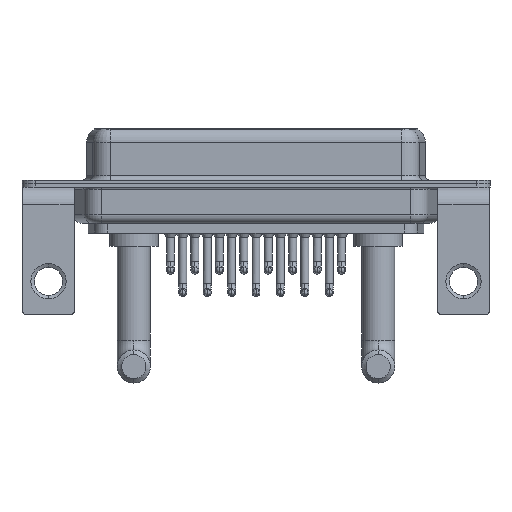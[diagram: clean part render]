
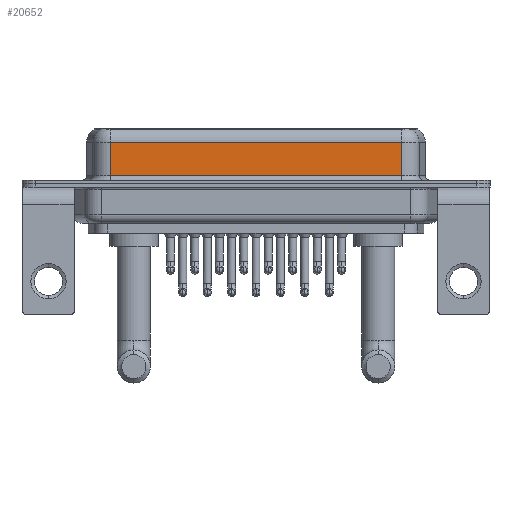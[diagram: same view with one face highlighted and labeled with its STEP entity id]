
A CAD part, front view. The second image highlights one B-rep face of the part: STEP entity #20652.
In plain terms, the highlighted planar face has unit normal (0, -1, 0).
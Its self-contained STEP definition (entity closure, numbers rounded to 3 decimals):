
#88 = DIRECTION ( 'NONE',  ( -1., 0., 0. ) ) ;
#593 = ORIENTED_EDGE ( 'NONE', *, *, #19188, .T. ) ;
#1705 = DIRECTION ( 'NONE',  ( 0., 0., -1. ) ) ;
#2007 = ORIENTED_EDGE ( 'NONE', *, *, #19016, .F. ) ;
#2986 = ORIENTED_EDGE ( 'NONE', *, *, #3895, .T. ) ;
#3107 = EDGE_CURVE ( 'NONE', #15258, #9774, #12984, .T. ) ;
#3604 = VERTEX_POINT ( 'NONE', #16222 ) ;
#3895 = EDGE_CURVE ( 'NONE', #4087, #15258, #15090, .T. ) ;
#4087 = VERTEX_POINT ( 'NONE', #20747 ) ;
#5536 = VECTOR ( 'NONE', #12917, 1000. ) ;
#6944 = VECTOR ( 'NONE', #18664, 1000. ) ;
#7232 = CARTESIAN_POINT ( 'NONE',  ( 7.013, -3.95, 4.65 ) ) ;
#7473 = AXIS2_PLACEMENT_3D ( 'NONE', #18118, #8065, #13878 ) ;
#8065 = DIRECTION ( 'NONE',  ( 0., 1., 0. ) ) ;
#8411 = CARTESIAN_POINT ( 'NONE',  ( 40.037, -3.95, 4.65 ) ) ;
#8516 = LINE ( 'NONE', #13898, #6944 ) ;
#9628 = LINE ( 'NONE', #14343, #5536 ) ;
#9713 = FACE_OUTER_BOUND ( 'NONE', #12321, .T. ) ;
#9774 = VERTEX_POINT ( 'NONE', #10964 ) ;
#10964 = CARTESIAN_POINT ( 'NONE',  ( 7.013, -3.95, 0.9 ) ) ;
#11774 = ORIENTED_EDGE ( 'NONE', *, *, #3107, .T. ) ;
#12321 = EDGE_LOOP ( 'NONE', ( #2007, #2986, #11774, #593 ) ) ;
#12917 = DIRECTION ( 'NONE',  ( 0., 0., -1. ) ) ;
#12984 = LINE ( 'NONE', #17994, #18425 ) ;
#13878 = DIRECTION ( 'NONE',  ( 0., 0., 1. ) ) ;
#13898 = CARTESIAN_POINT ( 'NONE',  ( 40.037, -3.95, 0.9 ) ) ;
#14343 = CARTESIAN_POINT ( 'NONE',  ( 40.037, -3.95, 6.4 ) ) ;
#15090 = LINE ( 'NONE', #8411, #15657 ) ;
#15258 = VERTEX_POINT ( 'NONE', #7232 ) ;
#15657 = VECTOR ( 'NONE', #88, 1000. ) ;
#16222 = CARTESIAN_POINT ( 'NONE',  ( 40.037, -3.95, 0.9 ) ) ;
#16377 = PLANE ( 'NONE',  #7473 ) ;
#17994 = CARTESIAN_POINT ( 'NONE',  ( 7.013, -3.95, 6.4 ) ) ;
#18118 = CARTESIAN_POINT ( 'NONE',  ( 40.037, -3.95, 6.4 ) ) ;
#18425 = VECTOR ( 'NONE', #1705, 1000. ) ;
#18664 = DIRECTION ( 'NONE',  ( 1., 0., 0. ) ) ;
#19016 = EDGE_CURVE ( 'NONE', #4087, #3604, #9628, .T. ) ;
#19188 = EDGE_CURVE ( 'NONE', #9774, #3604, #8516, .T. ) ;
#20652 = ADVANCED_FACE ( 'NONE', ( #9713 ), #16377, .F. ) ;
#20747 = CARTESIAN_POINT ( 'NONE',  ( 40.037, -3.95, 4.65 ) ) ;
